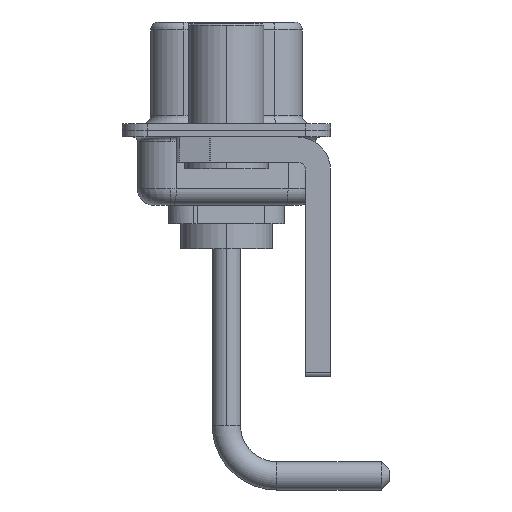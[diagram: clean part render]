
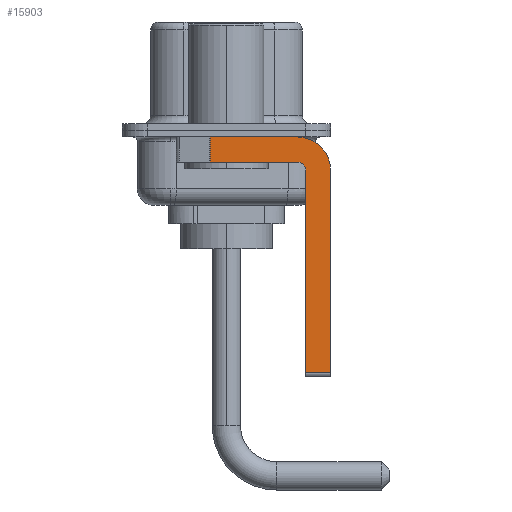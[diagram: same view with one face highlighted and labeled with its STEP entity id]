
A CAD part, left-side view. The second image highlights one B-rep face of the part: STEP entity #15903.
In plain terms, the highlighted planar face has unit normal (-1, 0, 0).
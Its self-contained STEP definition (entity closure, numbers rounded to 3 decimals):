
#399 = ORIENTED_EDGE ( 'NONE', *, *, #5888, .F. ) ;
#944 = LINE ( 'NONE', #2456, #12686 ) ;
#1012 = CARTESIAN_POINT ( 'NONE',  ( -2.9, -4.75, -2.4 ) ) ;
#1461 = VERTEX_POINT ( 'NONE', #4950 ) ;
#1514 = AXIS2_PLACEMENT_3D ( 'NONE', #13701, #12383, #6743 ) ;
#1962 = DIRECTION ( 'NONE',  ( 1., 0., 0. ) ) ;
#2009 = CARTESIAN_POINT ( 'NONE',  ( -2.9, 0.978, -0.4 ) ) ;
#2073 = CARTESIAN_POINT ( 'NONE',  ( -2.9, 0.978, -1.9 ) ) ;
#2147 = ORIENTED_EDGE ( 'NONE', *, *, #17000, .T. ) ;
#2456 = CARTESIAN_POINT ( 'NONE',  ( -2.9, -4.25, -14.55 ) ) ;
#2719 = EDGE_CURVE ( 'NONE', #13633, #4278, #10692, .T. ) ;
#2822 = EDGE_CURVE ( 'NONE', #7375, #4278, #17948, .T. ) ;
#2830 = CARTESIAN_POINT ( 'NONE',  ( -2.9, -6.25, -14.55 ) ) ;
#3237 = LINE ( 'NONE', #17609, #16598 ) ;
#3675 = LINE ( 'NONE', #10606, #12658 ) ;
#4066 = VECTOR ( 'NONE', #6197, 1000. ) ;
#4278 = VERTEX_POINT ( 'NONE', #2073 ) ;
#4601 = FACE_OUTER_BOUND ( 'NONE', #4966, .T. ) ;
#4872 = DIRECTION ( 'NONE',  ( 0., 0., -1. ) ) ;
#4926 = CARTESIAN_POINT ( 'NONE',  ( -2.9, -4.75, -14.55 ) ) ;
#4950 = CARTESIAN_POINT ( 'NONE',  ( -2.9, -4.25, -0.4 ) ) ;
#4966 = EDGE_LOOP ( 'NONE', ( #16523, #8882, #7503, #14026, #16765, #2147, #5736, #399 ) ) ;
#5339 = AXIS2_PLACEMENT_3D ( 'NONE', #11173, #9760, #9942 ) ;
#5736 = ORIENTED_EDGE ( 'NONE', *, *, #10295, .F. ) ;
#5888 = EDGE_CURVE ( 'NONE', #1461, #18556, #17043, .T. ) ;
#6197 = DIRECTION ( 'NONE',  ( 0., 0., -1. ) ) ;
#6698 = DIRECTION ( 'NONE',  ( 0., 0., -1. ) ) ;
#6743 = DIRECTION ( 'NONE',  ( 0., 0., 1. ) ) ;
#6953 = AXIS2_PLACEMENT_3D ( 'NONE', #17562, #1962, #4872 ) ;
#7375 = VERTEX_POINT ( 'NONE', #8807 ) ;
#7503 = ORIENTED_EDGE ( 'NONE', *, *, #2822, .F. ) ;
#7632 = VERTEX_POINT ( 'NONE', #1012 ) ;
#8102 = CARTESIAN_POINT ( 'NONE',  ( -2.9, -6.25, -2.4 ) ) ;
#8159 = DIRECTION ( 'NONE',  ( 0., -1., 0. ) ) ;
#8172 = VERTEX_POINT ( 'NONE', #2830 ) ;
#8433 = EDGE_CURVE ( 'NONE', #7632, #7375, #16211, .T. ) ;
#8807 = CARTESIAN_POINT ( 'NONE',  ( -2.9, -4.25, -1.9 ) ) ;
#8882 = ORIENTED_EDGE ( 'NONE', *, *, #2719, .T. ) ;
#9190 = CARTESIAN_POINT ( 'NONE',  ( -2.9, 0.978, -1.9 ) ) ;
#9227 = DIRECTION ( 'NONE',  ( 0., -1., 0. ) ) ;
#9760 = DIRECTION ( 'NONE',  ( 1., 0., 0. ) ) ;
#9872 = LINE ( 'NONE', #8102, #17773 ) ;
#9942 = DIRECTION ( 'NONE',  ( 0., 0., -1. ) ) ;
#10044 = VERTEX_POINT ( 'NONE', #4926 ) ;
#10295 = EDGE_CURVE ( 'NONE', #18556, #8172, #9872, .T. ) ;
#10606 = CARTESIAN_POINT ( 'NONE',  ( -2.9, -4.75, -14.8 ) ) ;
#10692 = LINE ( 'NONE', #9190, #4066 ) ;
#11173 = CARTESIAN_POINT ( 'NONE',  ( -2.9, -4.25, -2.4 ) ) ;
#12383 = DIRECTION ( 'NONE',  ( -1., 0., 0. ) ) ;
#12658 = VECTOR ( 'NONE', #14945, 1000. ) ;
#12686 = VECTOR ( 'NONE', #8159, 1000. ) ;
#13633 = VERTEX_POINT ( 'NONE', #2009 ) ;
#13701 = CARTESIAN_POINT ( 'NONE',  ( -2.9, -4.25, -2.4 ) ) ;
#14026 = ORIENTED_EDGE ( 'NONE', *, *, #8433, .F. ) ;
#14255 = EDGE_CURVE ( 'NONE', #10044, #7632, #3675, .T. ) ;
#14450 = PLANE ( 'NONE',  #6953 ) ;
#14856 = VECTOR ( 'NONE', #15213, 1000. ) ;
#14945 = DIRECTION ( 'NONE',  ( 0., 0., 1. ) ) ;
#14973 = EDGE_CURVE ( 'NONE', #13633, #1461, #3237, .T. ) ;
#15213 = DIRECTION ( 'NONE',  ( 0., 1., 0. ) ) ;
#15903 = ADVANCED_FACE ( 'NONE', ( #4601 ), #14450, .F. ) ;
#16211 = CIRCLE ( 'NONE', #1514, 0.5 ) ;
#16523 = ORIENTED_EDGE ( 'NONE', *, *, #14973, .F. ) ;
#16598 = VECTOR ( 'NONE', #9227, 1000. ) ;
#16765 = ORIENTED_EDGE ( 'NONE', *, *, #14255, .F. ) ;
#17000 = EDGE_CURVE ( 'NONE', #10044, #8172, #944, .T. ) ;
#17043 = CIRCLE ( 'NONE', #5339, 2. ) ;
#17254 = CARTESIAN_POINT ( 'NONE',  ( -2.9, -6.25, -2.4 ) ) ;
#17562 = CARTESIAN_POINT ( 'NONE',  ( -2.9, -4.25, -2.4 ) ) ;
#17609 = CARTESIAN_POINT ( 'NONE',  ( -2.9, 3., -0.4 ) ) ;
#17773 = VECTOR ( 'NONE', #6698, 1000. ) ;
#17850 = CARTESIAN_POINT ( 'NONE',  ( -2.9, -4.25, -1.9 ) ) ;
#17948 = LINE ( 'NONE', #17850, #14856 ) ;
#18556 = VERTEX_POINT ( 'NONE', #17254 ) ;
